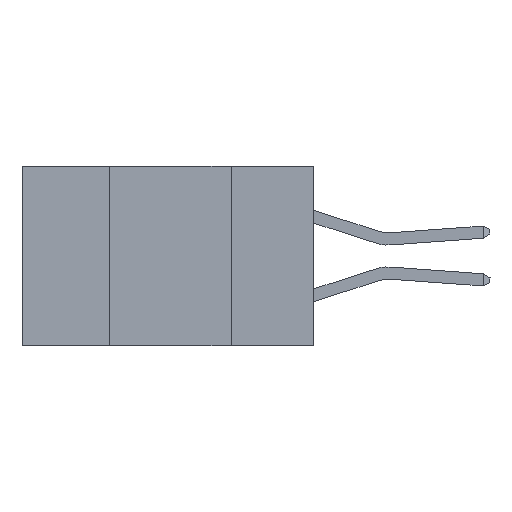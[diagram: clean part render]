
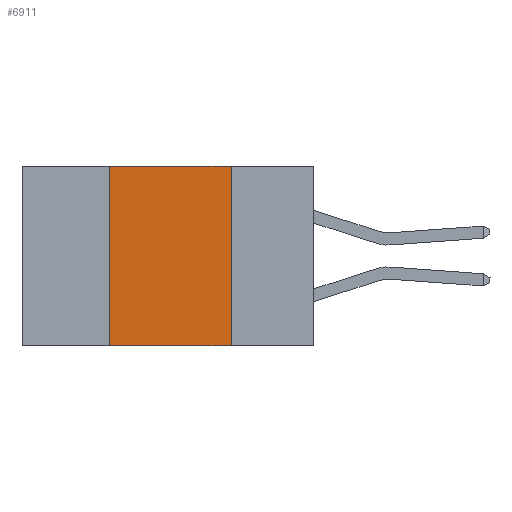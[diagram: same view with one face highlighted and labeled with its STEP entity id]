
A CAD part, left-side view. The second image highlights one B-rep face of the part: STEP entity #6911.
In plain terms, the highlighted planar face has unit normal (-1, 0, 0).
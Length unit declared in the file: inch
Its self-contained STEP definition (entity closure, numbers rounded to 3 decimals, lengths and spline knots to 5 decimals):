
#321 = VERTEX_POINT ( 'NONE', #15188 ) ;
#380 = VECTOR ( 'NONE', #12862, 39.37008 ) ;
#1191 = CARTESIAN_POINT ( 'NONE',  ( 0., 0.17, 0. ) ) ;
#1430 = VECTOR ( 'NONE', #15751, 39.37008 ) ;
#3114 = FACE_OUTER_BOUND ( 'NONE', #17277, .T. ) ;
#3660 = PLANE ( 'NONE',  #4505 ) ;
#4505 = AXIS2_PLACEMENT_3D ( 'NONE', #15498, #6690, #16919 ) ;
#4675 = LINE ( 'NONE', #15783, #380 ) ;
#5152 = ORIENTED_EDGE ( 'NONE', *, *, #7673, .F. ) ;
#5659 = VECTOR ( 'NONE', #9719, 39.37008 ) ;
#5825 = ORIENTED_EDGE ( 'NONE', *, *, #6952, .F. ) ;
#5937 = VERTEX_POINT ( 'NONE', #7099 ) ;
#6690 = DIRECTION ( 'NONE',  ( 1., 0., 0. ) ) ;
#6911 = ADVANCED_FACE ( 'NONE', ( #3114 ), #3660, .F. ) ;
#6952 = EDGE_CURVE ( 'NONE', #14503, #7748, #17364, .T. ) ;
#7099 = CARTESIAN_POINT ( 'NONE',  ( 0., 0.17, -0.37 ) ) ;
#7673 = EDGE_CURVE ( 'NONE', #321, #14503, #16859, .T. ) ;
#7748 = VERTEX_POINT ( 'NONE', #1191 ) ;
#8412 = CARTESIAN_POINT ( 'NONE',  ( 0., 0.6, -0.37 ) ) ;
#8729 = ORIENTED_EDGE ( 'NONE', *, *, #12006, .T. ) ;
#9094 = VECTOR ( 'NONE', #17083, 39.37008 ) ;
#9568 = ORIENTED_EDGE ( 'NONE', *, *, #16535, .F. ) ;
#9719 = DIRECTION ( 'NONE',  ( 0., -1., 0. ) ) ;
#9814 = CARTESIAN_POINT ( 'NONE',  ( 0., 0.42, 0. ) ) ;
#12006 = EDGE_CURVE ( 'NONE', #321, #5937, #17015, .T. ) ;
#12642 = CARTESIAN_POINT ( 'NONE',  ( 0., 0.6, 0. ) ) ;
#12862 = DIRECTION ( 'NONE',  ( 0., 0., -1. ) ) ;
#14503 = VERTEX_POINT ( 'NONE', #16107 ) ;
#15188 = CARTESIAN_POINT ( 'NONE',  ( 0., 0.42, -0.37 ) ) ;
#15498 = CARTESIAN_POINT ( 'NONE',  ( 0., 0.6, 0. ) ) ;
#15751 = DIRECTION ( 'NONE',  ( 0., -1., 0. ) ) ;
#15783 = CARTESIAN_POINT ( 'NONE',  ( 0., 0.17, 0. ) ) ;
#16107 = CARTESIAN_POINT ( 'NONE',  ( 0., 0.42, 0. ) ) ;
#16535 = EDGE_CURVE ( 'NONE', #7748, #5937, #4675, .T. ) ;
#16859 = LINE ( 'NONE', #9814, #9094 ) ;
#16919 = DIRECTION ( 'NONE',  ( 0., 0., -1. ) ) ;
#17015 = LINE ( 'NONE', #8412, #1430 ) ;
#17083 = DIRECTION ( 'NONE',  ( 0., 0., 1. ) ) ;
#17277 = EDGE_LOOP ( 'NONE', ( #9568, #5825, #5152, #8729 ) ) ;
#17364 = LINE ( 'NONE', #12642, #5659 ) ;
